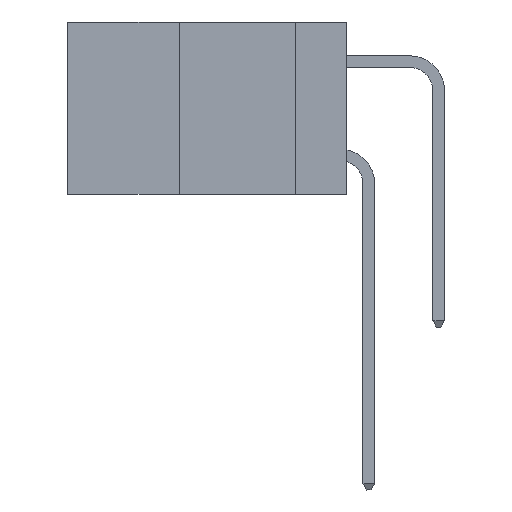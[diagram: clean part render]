
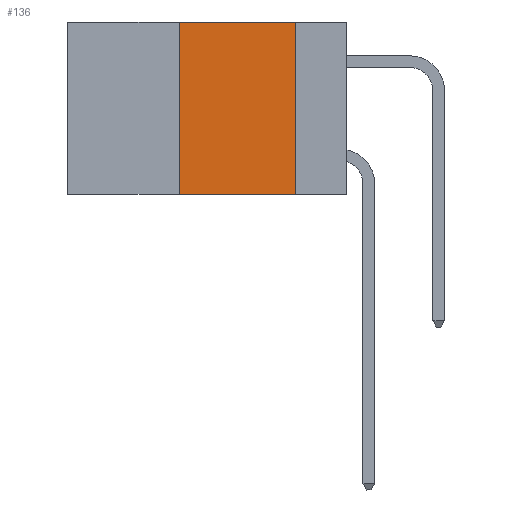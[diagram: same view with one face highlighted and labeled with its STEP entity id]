
A CAD part, left-side view. The second image highlights one B-rep face of the part: STEP entity #136.
In plain terms, the highlighted planar face has unit normal (-1, 0, 0).
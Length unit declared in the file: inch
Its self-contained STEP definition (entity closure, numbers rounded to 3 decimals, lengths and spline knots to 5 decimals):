
#66 = LINE ( 'NONE', #487, #12093 ) ;
#136 = ADVANCED_FACE ( 'NONE', ( #13571 ), #892, .F. ) ;
#487 = CARTESIAN_POINT ( 'NONE',  ( 0., 0.6, 0. ) ) ;
#759 = CARTESIAN_POINT ( 'NONE',  ( 0., 0.11, 0. ) ) ;
#892 = PLANE ( 'NONE',  #10742 ) ;
#1059 = EDGE_LOOP ( 'NONE', ( #8491, #4121, #7871, #8462 ) ) ;
#1768 = EDGE_CURVE ( 'NONE', #9066, #10212, #13135, .T. ) ;
#2600 = EDGE_CURVE ( 'NONE', #10212, #7279, #66, .T. ) ;
#2907 = CARTESIAN_POINT ( 'NONE',  ( 0., 0.36, 0. ) ) ;
#3506 = VECTOR ( 'NONE', #9387, 39.37008 ) ;
#3951 = CARTESIAN_POINT ( 'NONE',  ( 0., 0.36, 0. ) ) ;
#4121 = ORIENTED_EDGE ( 'NONE', *, *, #2600, .F. ) ;
#4853 = EDGE_CURVE ( 'NONE', #7279, #8727, #13928, .T. ) ;
#4975 = CARTESIAN_POINT ( 'NONE',  ( 0., 0.6, -0.37 ) ) ;
#7244 = LINE ( 'NONE', #4975, #3506 ) ;
#7279 = VERTEX_POINT ( 'NONE', #7957 ) ;
#7608 = VECTOR ( 'NONE', #12236, 39.37008 ) ;
#7871 = ORIENTED_EDGE ( 'NONE', *, *, #1768, .F. ) ;
#7957 = CARTESIAN_POINT ( 'NONE',  ( 0., 0.11, 0. ) ) ;
#8462 = ORIENTED_EDGE ( 'NONE', *, *, #9588, .T. ) ;
#8491 = ORIENTED_EDGE ( 'NONE', *, *, #4853, .F. ) ;
#8727 = VERTEX_POINT ( 'NONE', #10632 ) ;
#9066 = VERTEX_POINT ( 'NONE', #13346 ) ;
#9299 = DIRECTION ( 'NONE',  ( 0., -1., 0. ) ) ;
#9387 = DIRECTION ( 'NONE',  ( 0., -1., 0. ) ) ;
#9588 = EDGE_CURVE ( 'NONE', #9066, #8727, #7244, .T. ) ;
#10212 = VERTEX_POINT ( 'NONE', #3951 ) ;
#10615 = VECTOR ( 'NONE', #11667, 39.37008 ) ;
#10632 = CARTESIAN_POINT ( 'NONE',  ( 0., 0.11, -0.37 ) ) ;
#10742 = AXIS2_PLACEMENT_3D ( 'NONE', #12162, #12451, #12479 ) ;
#11667 = DIRECTION ( 'NONE',  ( 0., 0., -1. ) ) ;
#12093 = VECTOR ( 'NONE', #9299, 39.37008 ) ;
#12162 = CARTESIAN_POINT ( 'NONE',  ( 0., 0.6, 0. ) ) ;
#12236 = DIRECTION ( 'NONE',  ( 0., 0., 1. ) ) ;
#12451 = DIRECTION ( 'NONE',  ( 1., 0., 0. ) ) ;
#12479 = DIRECTION ( 'NONE',  ( 0., 0., -1. ) ) ;
#13135 = LINE ( 'NONE', #2907, #7608 ) ;
#13346 = CARTESIAN_POINT ( 'NONE',  ( 0., 0.36, -0.37 ) ) ;
#13571 = FACE_OUTER_BOUND ( 'NONE', #1059, .T. ) ;
#13928 = LINE ( 'NONE', #759, #10615 ) ;
